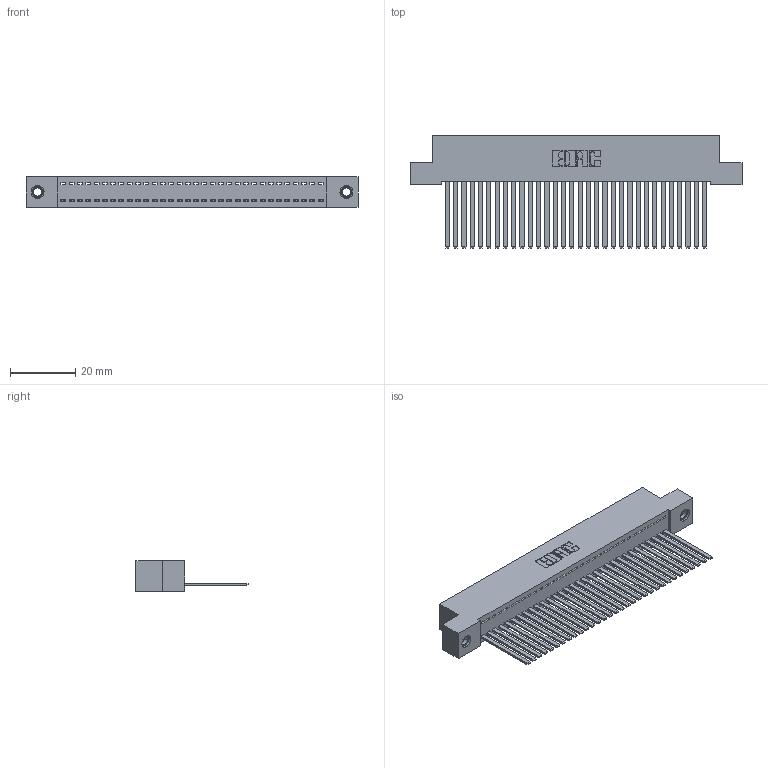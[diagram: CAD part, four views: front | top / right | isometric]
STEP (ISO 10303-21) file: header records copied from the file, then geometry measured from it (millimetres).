
FILE_DESCRIPTION (( 'STEP AP203' ), '1' );
FILE_NAME ('392-032-544-107.STEP', '2018-08-16T00:12:37', ( '' ), ( '' ), 'SwSTEP 2.0', 'SolidWorks 2016', '' );
FILE_SCHEMA (( 'CONFIG_CONTROL_DESIGN' ));
Length unit declared in the file: inch
Products named in the file (4): 345-292-001_345-293-144; 345-250-001_345-250-005-103; 392-032-544-107; 342 Part_TI
Assembly tree (35 placements, depth 2):
  392-032-544-107
    342 Part_TI
    345-292-001_345-293-144  x32
    345-250-001_345-250-005-103  x2
Bounding box: 101.6 x 34.3 x 9.4 mm (x, y, z)
Volume: 9229.4 mm3; surface area: 14453.2 mm2
Topology: 35 solids, 35 shells, 1834 faces, 5491 edges, 3610 vertices
Faces by surface type: plane 1314, cylinder 504, cone 12, torus 4
Entity records: 21726 total; most frequent: CARTESIAN_POINT 3729, ORIENTED_EDGE 3690, DIRECTION 3195, EDGE_CURVE 1845, VECTOR 1701, LINE 1701, VERTEX_POINT 1224, AXIS2_PLACEMENT_3D 747
